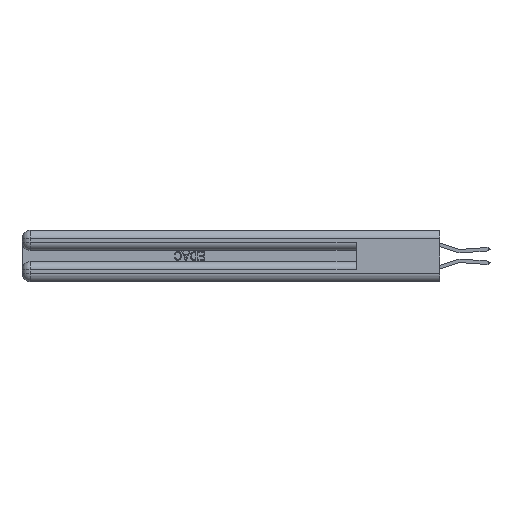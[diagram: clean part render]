
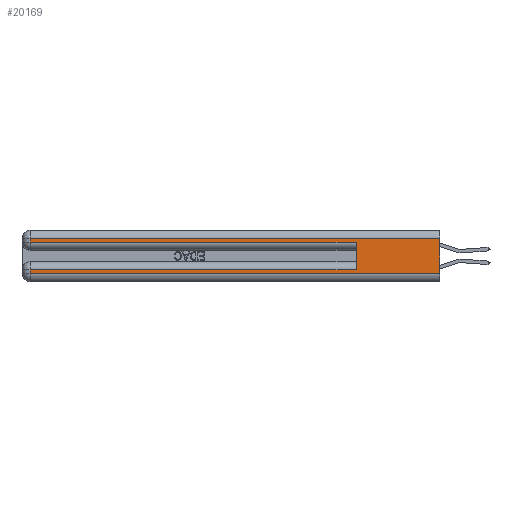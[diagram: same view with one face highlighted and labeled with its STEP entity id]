
A CAD part, left-side view. The second image highlights one B-rep face of the part: STEP entity #20169.
In plain terms, the highlighted planar face has unit normal (-1, 0, 0).
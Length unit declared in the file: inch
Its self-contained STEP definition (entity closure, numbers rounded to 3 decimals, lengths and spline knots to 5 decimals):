
#174 = DIRECTION ( 'NONE',  ( 0., 0., -1. ) ) ;
#527 = DIRECTION ( 'NONE',  ( 0., -1., 0. ) ) ;
#554 = CARTESIAN_POINT ( 'NONE',  ( 0., 2.94, 0.06 ) ) ;
#700 = ORIENTED_EDGE ( 'NONE', *, *, #42423, .T. ) ;
#831 = ORIENTED_EDGE ( 'NONE', *, *, #32846, .T. ) ;
#1177 = DIRECTION ( 'NONE',  ( 0., 0., -1. ) ) ;
#2214 = LINE ( 'NONE', #27043, #36281 ) ;
#2427 = LINE ( 'NONE', #13590, #36487 ) ;
#2882 = VERTEX_POINT ( 'NONE', #7033 ) ;
#3477 = CARTESIAN_POINT ( 'NONE',  ( 0., 2.94, 0.37 ) ) ;
#3952 = FACE_OUTER_BOUND ( 'NONE', #24510, .T. ) ;
#4357 = ORIENTED_EDGE ( 'NONE', *, *, #10759, .F. ) ;
#4512 = CARTESIAN_POINT ( 'NONE',  ( 0., 0., 0.06 ) ) ;
#6957 = CARTESIAN_POINT ( 'NONE',  ( 0., 2.94, 0.085 ) ) ;
#7033 = CARTESIAN_POINT ( 'NONE',  ( 0., 0.6, 0.085 ) ) ;
#7165 = VECTOR ( 'NONE', #31276, 39.37008 ) ;
#7761 = CARTESIAN_POINT ( 'NONE',  ( 0., 2.94, 0.31 ) ) ;
#8240 = CARTESIAN_POINT ( 'NONE',  ( 0., 0., 0.31 ) ) ;
#8523 = CARTESIAN_POINT ( 'NONE',  ( 0., 2.94, 0.285 ) ) ;
#8778 = ORIENTED_EDGE ( 'NONE', *, *, #38026, .T. ) ;
#10336 = LINE ( 'NONE', #35107, #18123 ) ;
#10617 = PLANE ( 'NONE',  #35373 ) ;
#10759 = EDGE_CURVE ( 'NONE', #2882, #41909, #41304, .T. ) ;
#10856 = DIRECTION ( 'NONE',  ( 0., 0., -1. ) ) ;
#11733 = LINE ( 'NONE', #21421, #42730 ) ;
#12985 = VERTEX_POINT ( 'NONE', #8240 ) ;
#13409 = LINE ( 'NONE', #3477, #33090 ) ;
#13590 = CARTESIAN_POINT ( 'NONE',  ( 0., 0., 0.06 ) ) ;
#13770 = DIRECTION ( 'NONE',  ( 0., 1., 0. ) ) ;
#14803 = ORIENTED_EDGE ( 'NONE', *, *, #15281, .T. ) ;
#15281 = EDGE_CURVE ( 'NONE', #39175, #41909, #24141, .T. ) ;
#16921 = EDGE_CURVE ( 'NONE', #12985, #23700, #2214, .T. ) ;
#17410 = VERTEX_POINT ( 'NONE', #6957 ) ;
#18123 = VECTOR ( 'NONE', #23027, 39.37008 ) ;
#18434 = EDGE_CURVE ( 'NONE', #2882, #17410, #10336, .T. ) ;
#20169 = ADVANCED_FACE ( 'NONE', ( #3952 ), #10617, .F. ) ;
#20334 = DIRECTION ( 'NONE',  ( 1., 0., 0. ) ) ;
#21421 = CARTESIAN_POINT ( 'NONE',  ( 0., 2.94, 0.37 ) ) ;
#22078 = VERTEX_POINT ( 'NONE', #554 ) ;
#23027 = DIRECTION ( 'NONE',  ( 0., 1., 0. ) ) ;
#23700 = VERTEX_POINT ( 'NONE', #7761 ) ;
#24091 = DIRECTION ( 'NONE',  ( 0., -1., 0. ) ) ;
#24141 = LINE ( 'NONE', #27134, #39570 ) ;
#24510 = EDGE_LOOP ( 'NONE', ( #35621, #40044, #831, #14803, #4357, #29859, #700, #8778 ) ) ;
#24945 = CARTESIAN_POINT ( 'NONE',  ( 0., 0.6, 0.145 ) ) ;
#27043 = CARTESIAN_POINT ( 'NONE',  ( 0., 0., 0.31 ) ) ;
#27134 = CARTESIAN_POINT ( 'NONE',  ( 0., 0., 0.285 ) ) ;
#29624 = VECTOR ( 'NONE', #10856, 39.37008 ) ;
#29859 = ORIENTED_EDGE ( 'NONE', *, *, #18434, .T. ) ;
#31276 = DIRECTION ( 'NONE',  ( 0., 0., 1. ) ) ;
#31969 = EDGE_CURVE ( 'NONE', #12985, #35102, #38876, .T. ) ;
#32846 = EDGE_CURVE ( 'NONE', #23700, #39175, #13409, .T. ) ;
#33090 = VECTOR ( 'NONE', #174, 39.37008 ) ;
#34274 = CARTESIAN_POINT ( 'NONE',  ( 0., 0., 0.37 ) ) ;
#35102 = VERTEX_POINT ( 'NONE', #4512 ) ;
#35107 = CARTESIAN_POINT ( 'NONE',  ( 0., 0., 0.085 ) ) ;
#35373 = AXIS2_PLACEMENT_3D ( 'NONE', #40197, #20334, #1177 ) ;
#35621 = ORIENTED_EDGE ( 'NONE', *, *, #31969, .F. ) ;
#36281 = VECTOR ( 'NONE', #13770, 39.37008 ) ;
#36487 = VECTOR ( 'NONE', #527, 39.37008 ) ;
#38026 = EDGE_CURVE ( 'NONE', #22078, #35102, #2427, .T. ) ;
#38876 = LINE ( 'NONE', #34274, #29624 ) ;
#39175 = VERTEX_POINT ( 'NONE', #8523 ) ;
#39570 = VECTOR ( 'NONE', #24091, 39.37008 ) ;
#40044 = ORIENTED_EDGE ( 'NONE', *, *, #16921, .T. ) ;
#40197 = CARTESIAN_POINT ( 'NONE',  ( 0., 0., 0.37 ) ) ;
#40887 = CARTESIAN_POINT ( 'NONE',  ( 0., 0.6, 0.285 ) ) ;
#41155 = DIRECTION ( 'NONE',  ( 0., 0., -1. ) ) ;
#41304 = LINE ( 'NONE', #24945, #7165 ) ;
#41909 = VERTEX_POINT ( 'NONE', #40887 ) ;
#42423 = EDGE_CURVE ( 'NONE', #17410, #22078, #11733, .T. ) ;
#42730 = VECTOR ( 'NONE', #41155, 39.37008 ) ;
